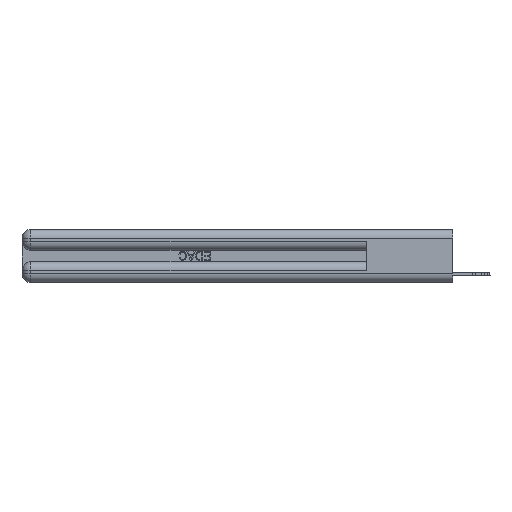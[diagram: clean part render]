
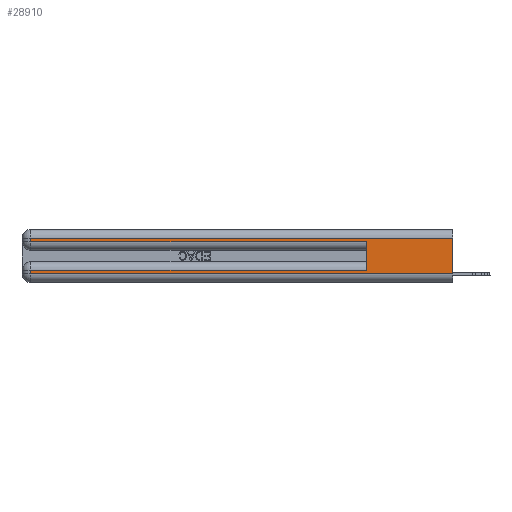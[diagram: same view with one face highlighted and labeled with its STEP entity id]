
A CAD part, left-side view. The second image highlights one B-rep face of the part: STEP entity #28910.
In plain terms, the highlighted planar face has unit normal (-1, 0, 0).
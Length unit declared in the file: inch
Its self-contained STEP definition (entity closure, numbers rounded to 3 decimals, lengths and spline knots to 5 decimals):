
#1097 = FACE_OUTER_BOUND ( 'NONE', #16551, .T. ) ;
#1330 = DIRECTION ( 'NONE',  ( 0., -1., 0. ) ) ;
#1403 = EDGE_CURVE ( 'NONE', #33051, #14633, #15388, .T. ) ;
#2001 = VERTEX_POINT ( 'NONE', #30740 ) ;
#2340 = EDGE_CURVE ( 'NONE', #2001, #7500, #8215, .T. ) ;
#3265 = LINE ( 'NONE', #18838, #23628 ) ;
#3496 = CARTESIAN_POINT ( 'NONE',  ( 0., 0., 0.06 ) ) ;
#4798 = LINE ( 'NONE', #27907, #30367 ) ;
#4898 = CARTESIAN_POINT ( 'NONE',  ( 0., 2.94, 0.085 ) ) ;
#5772 = CARTESIAN_POINT ( 'NONE',  ( 0., 0.6, 0.145 ) ) ;
#5786 = ORIENTED_EDGE ( 'NONE', *, *, #17287, .T. ) ;
#6098 = ORIENTED_EDGE ( 'NONE', *, *, #6683, .F. ) ;
#6423 = CARTESIAN_POINT ( 'NONE',  ( 0., 0., 0.37 ) ) ;
#6683 = EDGE_CURVE ( 'NONE', #22038, #7500, #13992, .T. ) ;
#7500 = VERTEX_POINT ( 'NONE', #30970 ) ;
#8215 = LINE ( 'NONE', #26307, #29615 ) ;
#9802 = ORIENTED_EDGE ( 'NONE', *, *, #19072, .T. ) ;
#10738 = DIRECTION ( 'NONE',  ( 0., 1., 0. ) ) ;
#11451 = LINE ( 'NONE', #6423, #27509 ) ;
#11627 = AXIS2_PLACEMENT_3D ( 'NONE', #14156, #16648, #11958 ) ;
#11958 = DIRECTION ( 'NONE',  ( 0., 0., -1. ) ) ;
#12717 = DIRECTION ( 'NONE',  ( 0., 0., -1. ) ) ;
#13493 = DIRECTION ( 'NONE',  ( 0., 0., -1. ) ) ;
#13758 = DIRECTION ( 'NONE',  ( 0., -1., 0. ) ) ;
#13992 = LINE ( 'NONE', #5772, #23975 ) ;
#14156 = CARTESIAN_POINT ( 'NONE',  ( 0., 0., 0.37 ) ) ;
#14488 = PLANE ( 'NONE',  #11627 ) ;
#14633 = VERTEX_POINT ( 'NONE', #17275 ) ;
#15388 = LINE ( 'NONE', #25602, #20942 ) ;
#15389 = EDGE_CURVE ( 'NONE', #17936, #2001, #3265, .T. ) ;
#15756 = CARTESIAN_POINT ( 'NONE',  ( 0., 0., 0.085 ) ) ;
#16551 = EDGE_LOOP ( 'NONE', ( #18574, #19373, #28291, #21839, #6098, #5786, #31664, #9802 ) ) ;
#16648 = DIRECTION ( 'NONE',  ( 1., 0., 0. ) ) ;
#17275 = CARTESIAN_POINT ( 'NONE',  ( 0., 2.94, 0.06 ) ) ;
#17287 = EDGE_CURVE ( 'NONE', #22038, #33051, #18288, .T. ) ;
#17524 = DIRECTION ( 'NONE',  ( 0., 1., 0. ) ) ;
#17936 = VERTEX_POINT ( 'NONE', #31609 ) ;
#18288 = LINE ( 'NONE', #15756, #18406 ) ;
#18404 = CARTESIAN_POINT ( 'NONE',  ( 0., 0., 0.31 ) ) ;
#18406 = VECTOR ( 'NONE', #10738, 39.37008 ) ;
#18422 = VECTOR ( 'NONE', #1330, 39.37008 ) ;
#18574 = ORIENTED_EDGE ( 'NONE', *, *, #23899, .F. ) ;
#18838 = CARTESIAN_POINT ( 'NONE',  ( 0., 2.94, 0.37 ) ) ;
#19001 = DIRECTION ( 'NONE',  ( 0., 0., 1. ) ) ;
#19072 = EDGE_CURVE ( 'NONE', #14633, #31985, #29262, .T. ) ;
#19373 = ORIENTED_EDGE ( 'NONE', *, *, #29799, .T. ) ;
#20942 = VECTOR ( 'NONE', #12717, 39.37008 ) ;
#21839 = ORIENTED_EDGE ( 'NONE', *, *, #2340, .T. ) ;
#22038 = VERTEX_POINT ( 'NONE', #30341 ) ;
#23628 = VECTOR ( 'NONE', #13493, 39.37008 ) ;
#23899 = EDGE_CURVE ( 'NONE', #31750, #31985, #11451, .T. ) ;
#23975 = VECTOR ( 'NONE', #19001, 39.37008 ) ;
#25602 = CARTESIAN_POINT ( 'NONE',  ( 0., 2.94, 0.37 ) ) ;
#26307 = CARTESIAN_POINT ( 'NONE',  ( 0., 0., 0.285 ) ) ;
#26858 = DIRECTION ( 'NONE',  ( 0., 0., -1. ) ) ;
#27509 = VECTOR ( 'NONE', #26858, 39.37008 ) ;
#27907 = CARTESIAN_POINT ( 'NONE',  ( 0., 0., 0.31 ) ) ;
#28291 = ORIENTED_EDGE ( 'NONE', *, *, #15389, .T. ) ;
#28910 = ADVANCED_FACE ( 'NONE', ( #1097 ), #14488, .F. ) ;
#29262 = LINE ( 'NONE', #3496, #18422 ) ;
#29615 = VECTOR ( 'NONE', #13758, 39.37008 ) ;
#29799 = EDGE_CURVE ( 'NONE', #31750, #17936, #4798, .T. ) ;
#30090 = CARTESIAN_POINT ( 'NONE',  ( 0., 0., 0.06 ) ) ;
#30341 = CARTESIAN_POINT ( 'NONE',  ( 0., 0.6, 0.085 ) ) ;
#30367 = VECTOR ( 'NONE', #17524, 39.37008 ) ;
#30740 = CARTESIAN_POINT ( 'NONE',  ( 0., 2.94, 0.285 ) ) ;
#30970 = CARTESIAN_POINT ( 'NONE',  ( 0., 0.6, 0.285 ) ) ;
#31609 = CARTESIAN_POINT ( 'NONE',  ( 0., 2.94, 0.31 ) ) ;
#31664 = ORIENTED_EDGE ( 'NONE', *, *, #1403, .T. ) ;
#31750 = VERTEX_POINT ( 'NONE', #18404 ) ;
#31985 = VERTEX_POINT ( 'NONE', #30090 ) ;
#33051 = VERTEX_POINT ( 'NONE', #4898 ) ;
